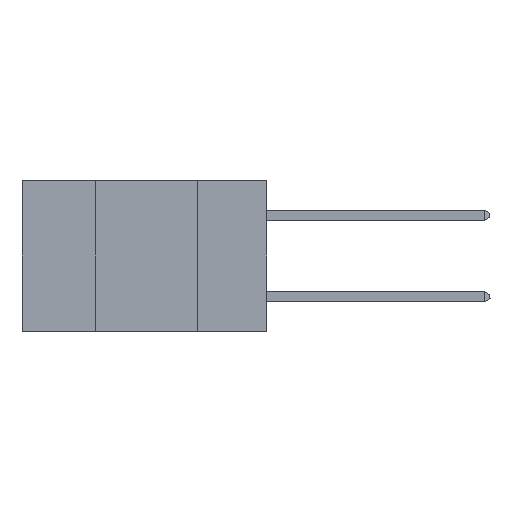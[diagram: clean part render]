
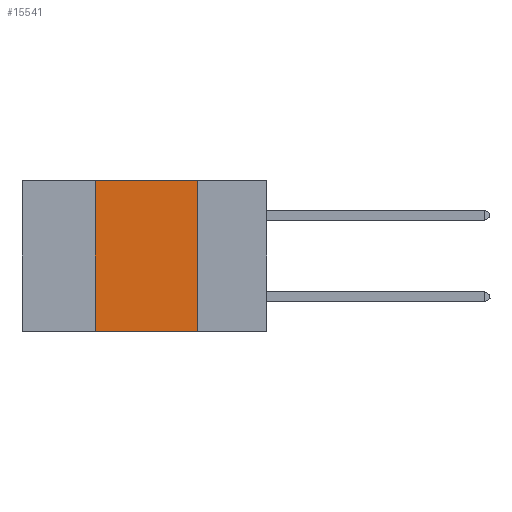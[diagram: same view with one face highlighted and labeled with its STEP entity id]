
A CAD part, left-side view. The second image highlights one B-rep face of the part: STEP entity #15541.
In plain terms, the highlighted planar face has unit normal (-1, 0, 0).
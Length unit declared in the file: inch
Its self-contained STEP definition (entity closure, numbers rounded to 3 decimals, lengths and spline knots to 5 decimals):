
#37 = VERTEX_POINT ( 'NONE', #8353 ) ;
#285 = LINE ( 'NONE', #13242, #17285 ) ;
#836 = CARTESIAN_POINT ( 'NONE',  ( 0., 0.42, 0. ) ) ;
#939 = LINE ( 'NONE', #6331, #16021 ) ;
#1459 = VERTEX_POINT ( 'NONE', #836 ) ;
#1710 = EDGE_LOOP ( 'NONE', ( #3762, #7312, #9586, #15584 ) ) ;
#2270 = PLANE ( 'NONE',  #14727 ) ;
#2374 = EDGE_CURVE ( 'NONE', #13905, #16362, #285, .T. ) ;
#3762 = ORIENTED_EDGE ( 'NONE', *, *, #2374, .F. ) ;
#4278 = VECTOR ( 'NONE', #6309, 39.37008 ) ;
#4679 = CARTESIAN_POINT ( 'NONE',  ( 0., 0.6, 0. ) ) ;
#4939 = DIRECTION ( 'NONE',  ( 0., 0., 1. ) ) ;
#5020 = DIRECTION ( 'NONE',  ( 0., 0., -1. ) ) ;
#5230 = EDGE_CURVE ( 'NONE', #1459, #13905, #8441, .T. ) ;
#5232 = CARTESIAN_POINT ( 'NONE',  ( 0., 0.6, 0. ) ) ;
#6309 = DIRECTION ( 'NONE',  ( 0., -1., 0. ) ) ;
#6331 = CARTESIAN_POINT ( 'NONE',  ( 0., 0.42, 0. ) ) ;
#7197 = EDGE_CURVE ( 'NONE', #37, #16362, #8634, .T. ) ;
#7312 = ORIENTED_EDGE ( 'NONE', *, *, #5230, .F. ) ;
#8353 = CARTESIAN_POINT ( 'NONE',  ( 0., 0.42, -0.37 ) ) ;
#8441 = LINE ( 'NONE', #4679, #9751 ) ;
#8567 = DIRECTION ( 'NONE',  ( 0., -1., 0. ) ) ;
#8634 = LINE ( 'NONE', #14746, #4278 ) ;
#9586 = ORIENTED_EDGE ( 'NONE', *, *, #15468, .F. ) ;
#9751 = VECTOR ( 'NONE', #8567, 39.37008 ) ;
#9996 = CARTESIAN_POINT ( 'NONE',  ( 0., 0.17, -0.37 ) ) ;
#10498 = CARTESIAN_POINT ( 'NONE',  ( 0., 0.17, 0. ) ) ;
#13242 = CARTESIAN_POINT ( 'NONE',  ( 0., 0.17, 0. ) ) ;
#13905 = VERTEX_POINT ( 'NONE', #10498 ) ;
#14727 = AXIS2_PLACEMENT_3D ( 'NONE', #5232, #16209, #16335 ) ;
#14746 = CARTESIAN_POINT ( 'NONE',  ( 0., 0.6, -0.37 ) ) ;
#15468 = EDGE_CURVE ( 'NONE', #37, #1459, #939, .T. ) ;
#15541 = ADVANCED_FACE ( 'NONE', ( #17102 ), #2270, .F. ) ;
#15584 = ORIENTED_EDGE ( 'NONE', *, *, #7197, .T. ) ;
#16021 = VECTOR ( 'NONE', #4939, 39.37008 ) ;
#16209 = DIRECTION ( 'NONE',  ( 1., 0., 0. ) ) ;
#16335 = DIRECTION ( 'NONE',  ( 0., 0., -1. ) ) ;
#16362 = VERTEX_POINT ( 'NONE', #9996 ) ;
#17102 = FACE_OUTER_BOUND ( 'NONE', #1710, .T. ) ;
#17285 = VECTOR ( 'NONE', #5020, 39.37008 ) ;
